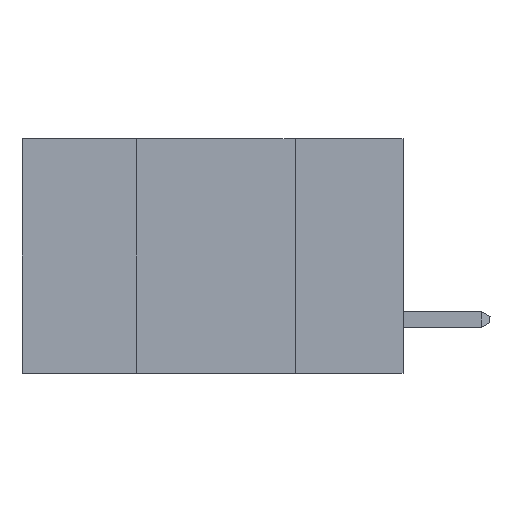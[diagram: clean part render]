
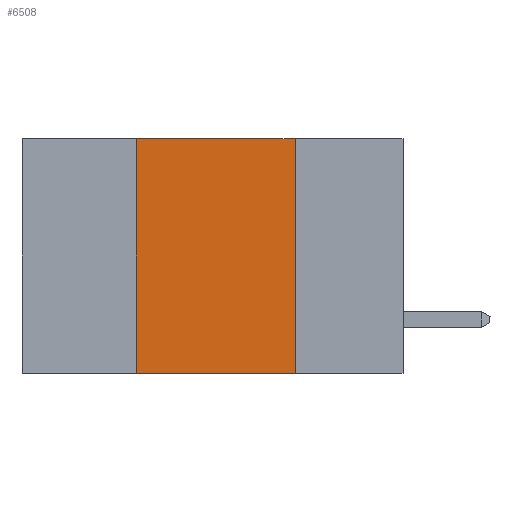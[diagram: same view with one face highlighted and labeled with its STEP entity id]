
A CAD part, left-side view. The second image highlights one B-rep face of the part: STEP entity #6508.
In plain terms, the highlighted planar face has unit normal (-1, 0, 0).
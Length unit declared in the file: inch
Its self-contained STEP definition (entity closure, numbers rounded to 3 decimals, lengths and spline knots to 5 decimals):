
#3 = LINE ( 'NONE', #19164, #10069 ) ;
#333 = CARTESIAN_POINT ( 'NONE',  ( 0., 0.17, 0. ) ) ;
#1049 = CARTESIAN_POINT ( 'NONE',  ( 0., 0.6, -0.37 ) ) ;
#1337 = DIRECTION ( 'NONE',  ( 0., -1., 0. ) ) ;
#1506 = LINE ( 'NONE', #333, #7797 ) ;
#1674 = VECTOR ( 'NONE', #11921, 39.37008 ) ;
#1799 = DIRECTION ( 'NONE',  ( 1., 0., 0. ) ) ;
#2990 = CARTESIAN_POINT ( 'NONE',  ( 0., 0.42, 0. ) ) ;
#4097 = VERTEX_POINT ( 'NONE', #8335 ) ;
#4991 = AXIS2_PLACEMENT_3D ( 'NONE', #15126, #1799, #13865 ) ;
#5797 = LINE ( 'NONE', #2990, #1674 ) ;
#6380 = EDGE_CURVE ( 'NONE', #7371, #7254, #1506, .T. ) ;
#6508 = ADVANCED_FACE ( 'NONE', ( #7934 ), #9193, .F. ) ;
#6517 = EDGE_LOOP ( 'NONE', ( #8300, #16362, #17861, #11196 ) ) ;
#7254 = VERTEX_POINT ( 'NONE', #18941 ) ;
#7371 = VERTEX_POINT ( 'NONE', #10666 ) ;
#7797 = VECTOR ( 'NONE', #18314, 39.37008 ) ;
#7934 = FACE_OUTER_BOUND ( 'NONE', #6517, .T. ) ;
#8300 = ORIENTED_EDGE ( 'NONE', *, *, #6380, .F. ) ;
#8335 = CARTESIAN_POINT ( 'NONE',  ( 0., 0.42, -0.37 ) ) ;
#9193 = PLANE ( 'NONE',  #4991 ) ;
#9327 = LINE ( 'NONE', #1049, #14131 ) ;
#10069 = VECTOR ( 'NONE', #11689, 39.37008 ) ;
#10666 = CARTESIAN_POINT ( 'NONE',  ( 0., 0.17, 0. ) ) ;
#11196 = ORIENTED_EDGE ( 'NONE', *, *, #16630, .T. ) ;
#11689 = DIRECTION ( 'NONE',  ( 0., -1., 0. ) ) ;
#11921 = DIRECTION ( 'NONE',  ( 0., 0., 1. ) ) ;
#13119 = EDGE_CURVE ( 'NONE', #4097, #16233, #5797, .T. ) ;
#13865 = DIRECTION ( 'NONE',  ( 0., 0., -1. ) ) ;
#14131 = VECTOR ( 'NONE', #1337, 39.37008 ) ;
#15126 = CARTESIAN_POINT ( 'NONE',  ( 0., 0.6, 0. ) ) ;
#16233 = VERTEX_POINT ( 'NONE', #19063 ) ;
#16362 = ORIENTED_EDGE ( 'NONE', *, *, #17599, .F. ) ;
#16630 = EDGE_CURVE ( 'NONE', #4097, #7254, #9327, .T. ) ;
#17599 = EDGE_CURVE ( 'NONE', #16233, #7371, #3, .T. ) ;
#17861 = ORIENTED_EDGE ( 'NONE', *, *, #13119, .F. ) ;
#18314 = DIRECTION ( 'NONE',  ( 0., 0., -1. ) ) ;
#18941 = CARTESIAN_POINT ( 'NONE',  ( 0., 0.17, -0.37 ) ) ;
#19063 = CARTESIAN_POINT ( 'NONE',  ( 0., 0.42, 0. ) ) ;
#19164 = CARTESIAN_POINT ( 'NONE',  ( 0., 0.6, 0. ) ) ;
